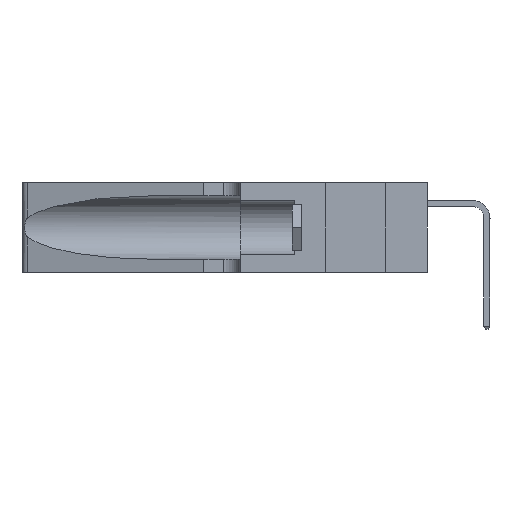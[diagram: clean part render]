
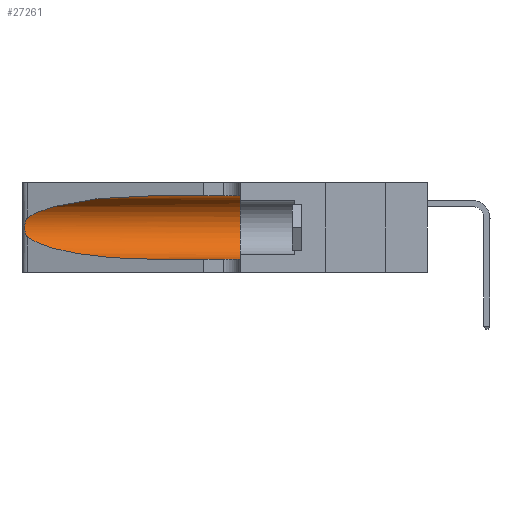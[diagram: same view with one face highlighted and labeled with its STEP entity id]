
A CAD part, left-side view. The second image highlights one B-rep face of the part: STEP entity #27261.
In plain terms, the highlighted cylindrical face has radius 3.308 mm (diameter 6.617 mm), a partial arc.
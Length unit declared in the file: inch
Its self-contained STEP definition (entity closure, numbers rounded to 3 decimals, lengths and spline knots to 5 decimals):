
#101 = EDGE_CURVE ( 'NONE', #8590, #21270, #5707, .T. ) ;
#724 = CARTESIAN_POINT ( 'NONE',  ( 0.2373, 1.15595, 0.08982 ) ) ;
#898 = EDGE_LOOP ( 'NONE', ( #9946, #27231, #21978, #25312, #25649, #7634 ) ) ;
#2330 = CARTESIAN_POINT ( 'NONE',  ( 0.1305, 0.35, 0.05475 ) ) ;
#4023 = VERTEX_POINT ( 'NONE', #2330 ) ;
#4159 = DIRECTION ( 'NONE',  ( 0., 1., 0. ) ) ;
#4177 = EDGE_CURVE ( 'NONE', #21270, #17439, #13620, .T. ) ;
#4280 = CARTESIAN_POINT ( 'NONE',  ( 0.25555, 1.22994, 0.2215 ) ) ;
#4304 = CARTESIAN_POINT ( 'NONE',  ( 0.26018, 1.23835, 0.19895 ) ) ;
#4375 = EDGE_CURVE ( 'NONE', #24797, #8590, #10548, .T. ) ;
#5288 = AXIS2_PLACEMENT_3D ( 'NONE', #23830, #11087, #25959 ) ;
#5368 = CARTESIAN_POINT ( 'NONE',  ( 0.1305, 0.35, 0.31525 ) ) ;
#5707 = B_SPLINE_CURVE_WITH_KNOTS ( 'NONE', 3,
 ( #21285, #4280, #18372, #14504, #14237, #4304, #12900, #12843, #18238, #18083, #18176, #9930, #7067, #6943 ),
 .UNSPECIFIED., .F., .F.,
 ( 4, 2, 2, 2, 2, 2, 4 ),
 ( 0., 0.00027, 0.00053, 0.00107, 0.0016, 0.00187, 0.00214 ),
 .UNSPECIFIED. ) ;
#6943 = CARTESIAN_POINT ( 'NONE',  ( 0.25487, 1.22718, 0.14631 ) ) ;
#7067 = CARTESIAN_POINT ( 'NONE',  ( 0.25555, 1.22993, 0.14849 ) ) ;
#7599 = CIRCLE ( 'NONE', #11153, 0.13025 ) ;
#7634 = ORIENTED_EDGE ( 'NONE', *, *, #21410, .F. ) ;
#7977 = LINE ( 'NONE', #15753, #24353 ) ;
#8067 = CARTESIAN_POINT ( 'NONE',  ( 0.1305, 1.61858, 0.31525 ) ) ;
#8513 = LINE ( 'NONE', #8067, #24211 ) ;
#8590 = VERTEX_POINT ( 'NONE', #19333 ) ;
#8736 = CARTESIAN_POINT ( 'NONE',  ( 0.1305, 0.72297, 0.31525 ) ) ;
#9440 = EDGE_CURVE ( 'NONE', #17439, #4023, #7977, .T. ) ;
#9807 = CARTESIAN_POINT ( 'NONE',  ( 0.25487, 1.22718, 0.14631 ) ) ;
#9930 = CARTESIAN_POINT ( 'NONE',  ( 0.25639, 1.23186, 0.15144 ) ) ;
#9946 = ORIENTED_EDGE ( 'NONE', *, *, #4375, .T. ) ;
#10157 = CARTESIAN_POINT ( 'NONE',  ( 0.18966, 0.96281, 0.31525 ) ) ;
#10548 =( BOUNDED_CURVE ( )  B_SPLINE_CURVE ( 3, ( #22915, #10157, #25022, #12293 ),
 .UNSPECIFIED., .F., .T. ) 
 B_SPLINE_CURVE_WITH_KNOTS ( ( 4, 4 ),
 ( 1.5708, 2.84003 ),
 .UNSPECIFIED. ) 
 CURVE ( )  GEOMETRIC_REPRESENTATION_ITEM ( )  RATIONAL_B_SPLINE_CURVE ( ( 1., 0.87, 0.87, 1. ) ) 
 REPRESENTATION_ITEM ( '' )  );
#11087 = DIRECTION ( 'NONE',  ( 0., -1., 0. ) ) ;
#11153 = AXIS2_PLACEMENT_3D ( 'NONE', #17065, #4159, #19222 ) ;
#11585 = VERTEX_POINT ( 'NONE', #5368 ) ;
#11652 = CARTESIAN_POINT ( 'NONE',  ( 0.1305, 0.72297, 0.05475 ) ) ;
#12293 = CARTESIAN_POINT ( 'NONE',  ( 0.25487, 1.22718, 0.22369 ) ) ;
#12843 = CARTESIAN_POINT ( 'NONE',  ( 0.26075, 1.23896, 0.178 ) ) ;
#12900 = CARTESIAN_POINT ( 'NONE',  ( 0.26075, 1.23896, 0.19203 ) ) ;
#13620 =( BOUNDED_CURVE ( )  B_SPLINE_CURVE ( 3, ( #13721, #724, #24396, #11652 ),
 .UNSPECIFIED., .F., .F. ) 
 B_SPLINE_CURVE_WITH_KNOTS ( ( 4, 4 ),
 ( 3.44316, 4.71239 ),
 .UNSPECIFIED. ) 
 CURVE ( )  GEOMETRIC_REPRESENTATION_ITEM ( )  RATIONAL_B_SPLINE_CURVE ( ( 1., 0.87, 0.87, 1. ) ) 
 REPRESENTATION_ITEM ( '' )  );
#13721 = CARTESIAN_POINT ( 'NONE',  ( 0.25487, 1.22718, 0.14631 ) ) ;
#14237 = CARTESIAN_POINT ( 'NONE',  ( 0.25854, 1.2359, 0.20912 ) ) ;
#14504 = CARTESIAN_POINT ( 'NONE',  ( 0.25787, 1.23484, 0.2124 ) ) ;
#15753 = CARTESIAN_POINT ( 'NONE',  ( 0.1305, 1.61858, 0.05475 ) ) ;
#16244 = CARTESIAN_POINT ( 'NONE',  ( 0.1305, 0.72297, 0.05475 ) ) ;
#17065 = CARTESIAN_POINT ( 'NONE',  ( 0.1305, 0.35, 0.185 ) ) ;
#17439 = VERTEX_POINT ( 'NONE', #16244 ) ;
#17896 = DIRECTION ( 'NONE',  ( 0., -1., 0. ) ) ;
#18083 = CARTESIAN_POINT ( 'NONE',  ( 0.25856, 1.23593, 0.16098 ) ) ;
#18176 = CARTESIAN_POINT ( 'NONE',  ( 0.25789, 1.23486, 0.15765 ) ) ;
#18238 = CARTESIAN_POINT ( 'NONE',  ( 0.26017, 1.23833, 0.17102 ) ) ;
#18372 = CARTESIAN_POINT ( 'NONE',  ( 0.25639, 1.23184, 0.21858 ) ) ;
#19019 = EDGE_CURVE ( 'NONE', #11585, #4023, #7599, .T. ) ;
#19222 = DIRECTION ( 'NONE',  ( 0., 0., 1. ) ) ;
#19333 = CARTESIAN_POINT ( 'NONE',  ( 0.25487, 1.22718, 0.22369 ) ) ;
#21270 = VERTEX_POINT ( 'NONE', #9807 ) ;
#21285 = CARTESIAN_POINT ( 'NONE',  ( 0.25487, 1.22718, 0.22369 ) ) ;
#21410 = EDGE_CURVE ( 'NONE', #24797, #11585, #8513, .T. ) ;
#21978 = ORIENTED_EDGE ( 'NONE', *, *, #4177, .T. ) ;
#22915 = CARTESIAN_POINT ( 'NONE',  ( 0.1305, 0.72297, 0.31525 ) ) ;
#23336 = CYLINDRICAL_SURFACE ( 'NONE', #5288, 0.13025 ) ;
#23830 = CARTESIAN_POINT ( 'NONE',  ( 0.1305, 1.61858, 0.185 ) ) ;
#23998 = FACE_OUTER_BOUND ( 'NONE', #898, .T. ) ;
#24211 = VECTOR ( 'NONE', #25136, 39.37008 ) ;
#24353 = VECTOR ( 'NONE', #17896, 39.37008 ) ;
#24396 = CARTESIAN_POINT ( 'NONE',  ( 0.18966, 0.96281, 0.05475 ) ) ;
#24797 = VERTEX_POINT ( 'NONE', #8736 ) ;
#25022 = CARTESIAN_POINT ( 'NONE',  ( 0.2373, 1.15595, 0.28018 ) ) ;
#25136 = DIRECTION ( 'NONE',  ( 0., -1., 0. ) ) ;
#25312 = ORIENTED_EDGE ( 'NONE', *, *, #9440, .T. ) ;
#25649 = ORIENTED_EDGE ( 'NONE', *, *, #19019, .F. ) ;
#25959 = DIRECTION ( 'NONE',  ( 0., 0., -1. ) ) ;
#27231 = ORIENTED_EDGE ( 'NONE', *, *, #101, .T. ) ;
#27261 = ADVANCED_FACE ( 'NONE', ( #23998 ), #23336, .F. ) ;
